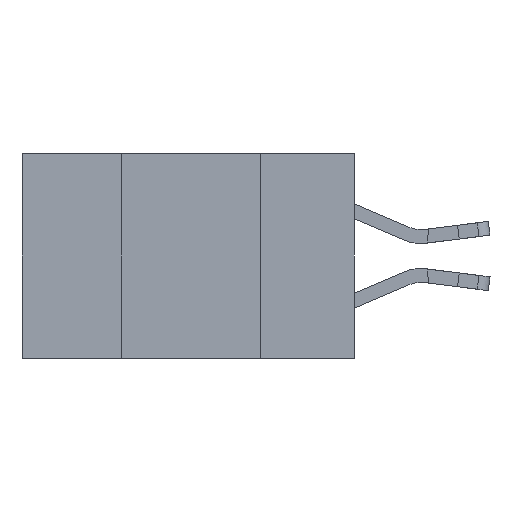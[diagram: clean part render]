
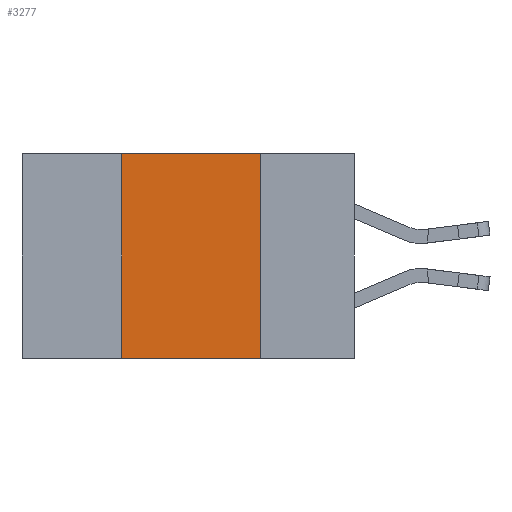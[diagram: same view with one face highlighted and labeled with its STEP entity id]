
A CAD part, left-side view. The second image highlights one B-rep face of the part: STEP entity #3277.
In plain terms, the highlighted planar face has unit normal (-1, 0, 0).
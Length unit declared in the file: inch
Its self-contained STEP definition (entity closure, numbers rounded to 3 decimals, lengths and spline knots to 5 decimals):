
#174 = CARTESIAN_POINT ( 'NONE',  ( 0., 0.6, 0. ) ) ;
#395 = EDGE_CURVE ( 'NONE', #9533, #8901, #4129, .T. ) ;
#1017 = VERTEX_POINT ( 'NONE', #2645 ) ;
#1469 = CARTESIAN_POINT ( 'NONE',  ( 0., 0.42, 0. ) ) ;
#2570 = VECTOR ( 'NONE', #9069, 39.37008 ) ;
#2622 = DIRECTION ( 'NONE',  ( 0., 0., -1. ) ) ;
#2642 = EDGE_CURVE ( 'NONE', #7099, #9533, #13041, .T. ) ;
#2645 = CARTESIAN_POINT ( 'NONE',  ( 0., 0.42, -0.37 ) ) ;
#2665 = DIRECTION ( 'NONE',  ( 1., 0., 0. ) ) ;
#3012 = ORIENTED_EDGE ( 'NONE', *, *, #5876, .F. ) ;
#3192 = PLANE ( 'NONE',  #11368 ) ;
#3277 = ADVANCED_FACE ( 'NONE', ( #8931 ), #3192, .F. ) ;
#3351 = EDGE_CURVE ( 'NONE', #1017, #8901, #12492, .T. ) ;
#3489 = CARTESIAN_POINT ( 'NONE',  ( 0., 0.6, 0. ) ) ;
#4129 = LINE ( 'NONE', #11971, #8869 ) ;
#4910 = DIRECTION ( 'NONE',  ( 0., 0., 1. ) ) ;
#5004 = CARTESIAN_POINT ( 'NONE',  ( 0., 0.42, -0.37 ) ) ;
#5818 = ORIENTED_EDGE ( 'NONE', *, *, #2642, .F. ) ;
#5876 = EDGE_CURVE ( 'NONE', #1017, #7099, #12741, .T. ) ;
#7099 = VERTEX_POINT ( 'NONE', #1469 ) ;
#7101 = ORIENTED_EDGE ( 'NONE', *, *, #3351, .T. ) ;
#7976 = CARTESIAN_POINT ( 'NONE',  ( 0., 0.17, -0.37 ) ) ;
#7995 = VECTOR ( 'NONE', #12413, 39.37008 ) ;
#8869 = VECTOR ( 'NONE', #11060, 39.37008 ) ;
#8901 = VERTEX_POINT ( 'NONE', #7976 ) ;
#8931 = FACE_OUTER_BOUND ( 'NONE', #9530, .T. ) ;
#9069 = DIRECTION ( 'NONE',  ( 0., -1., 0. ) ) ;
#9121 = ORIENTED_EDGE ( 'NONE', *, *, #395, .F. ) ;
#9530 = EDGE_LOOP ( 'NONE', ( #9121, #5818, #3012, #7101 ) ) ;
#9533 = VERTEX_POINT ( 'NONE', #11023 ) ;
#9620 = CARTESIAN_POINT ( 'NONE',  ( 0., 0.6, -0.37 ) ) ;
#9976 = VECTOR ( 'NONE', #4910, 39.37008 ) ;
#11023 = CARTESIAN_POINT ( 'NONE',  ( 0., 0.17, 0. ) ) ;
#11060 = DIRECTION ( 'NONE',  ( 0., 0., -1. ) ) ;
#11368 = AXIS2_PLACEMENT_3D ( 'NONE', #3489, #2665, #2622 ) ;
#11971 = CARTESIAN_POINT ( 'NONE',  ( 0., 0.17, -0.37 ) ) ;
#12413 = DIRECTION ( 'NONE',  ( 0., -1., 0. ) ) ;
#12492 = LINE ( 'NONE', #9620, #2570 ) ;
#12741 = LINE ( 'NONE', #5004, #9976 ) ;
#13041 = LINE ( 'NONE', #174, #7995 ) ;
